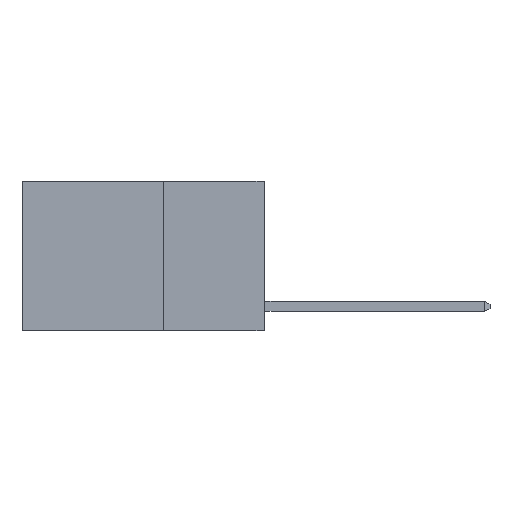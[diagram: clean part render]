
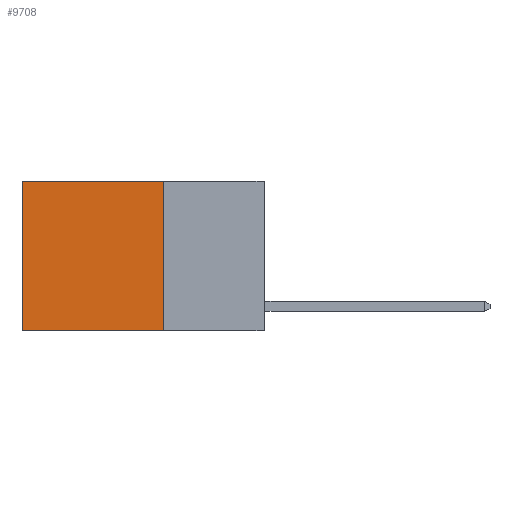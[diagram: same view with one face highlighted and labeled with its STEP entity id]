
A CAD part, left-side view. The second image highlights one B-rep face of the part: STEP entity #9708.
In plain terms, the highlighted planar face has unit normal (-1, 0, 0).
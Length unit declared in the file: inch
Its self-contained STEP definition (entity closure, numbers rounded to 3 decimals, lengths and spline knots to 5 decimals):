
#204 = EDGE_LOOP ( 'NONE', ( #6162, #4687, #380, #394 ) ) ;
#275 = AXIS2_PLACEMENT_3D ( 'NONE', #8043, #2861, #8905 ) ;
#380 = ORIENTED_EDGE ( 'NONE', *, *, #5318, .F. ) ;
#394 = ORIENTED_EDGE ( 'NONE', *, *, #443, .T. ) ;
#443 = EDGE_CURVE ( 'NONE', #10742, #9197, #7298, .T. ) ;
#632 = EDGE_CURVE ( 'NONE', #9197, #9472, #6686, .T. ) ;
#755 = CARTESIAN_POINT ( 'NONE',  ( 0.2625, 0.25, -0.37 ) ) ;
#899 = CARTESIAN_POINT ( 'NONE',  ( 0.2625, 0.6, 0. ) ) ;
#1655 = CARTESIAN_POINT ( 'NONE',  ( 0.2625, 0.6, -0.37 ) ) ;
#2075 = DIRECTION ( 'NONE',  ( 0., 1., 0. ) ) ;
#2601 = CARTESIAN_POINT ( 'NONE',  ( 0.2625, 0.25, 0. ) ) ;
#2861 = DIRECTION ( 'NONE',  ( 1., 0., 0. ) ) ;
#4158 = VECTOR ( 'NONE', #10157, 39.37008 ) ;
#4687 = ORIENTED_EDGE ( 'NONE', *, *, #9145, .F. ) ;
#5124 = LINE ( 'NONE', #2601, #9412 ) ;
#5318 = EDGE_CURVE ( 'NONE', #10742, #5752, #5124, .T. ) ;
#5542 = CARTESIAN_POINT ( 'NONE',  ( 0.2625, 0.25, -0.37 ) ) ;
#5752 = VERTEX_POINT ( 'NONE', #755 ) ;
#6101 = DIRECTION ( 'NONE',  ( 0., 0., -1. ) ) ;
#6162 = ORIENTED_EDGE ( 'NONE', *, *, #632, .T. ) ;
#6234 = CARTESIAN_POINT ( 'NONE',  ( 0.2625, 0.25, 0. ) ) ;
#6686 = LINE ( 'NONE', #899, #11006 ) ;
#7283 = VECTOR ( 'NONE', #2075, 39.37008 ) ;
#7298 = LINE ( 'NONE', #11034, #4158 ) ;
#7403 = FACE_OUTER_BOUND ( 'NONE', #204, .T. ) ;
#8043 = CARTESIAN_POINT ( 'NONE',  ( 0.2625, 0.25, 0. ) ) ;
#8905 = DIRECTION ( 'NONE',  ( 0., 0., -1. ) ) ;
#9145 = EDGE_CURVE ( 'NONE', #5752, #9472, #9290, .T. ) ;
#9197 = VERTEX_POINT ( 'NONE', #9906 ) ;
#9290 = LINE ( 'NONE', #5542, #7283 ) ;
#9412 = VECTOR ( 'NONE', #11256, 39.37008 ) ;
#9472 = VERTEX_POINT ( 'NONE', #1655 ) ;
#9708 = ADVANCED_FACE ( 'NONE', ( #7403 ), #10609, .F. ) ;
#9906 = CARTESIAN_POINT ( 'NONE',  ( 0.2625, 0.6, 0. ) ) ;
#10157 = DIRECTION ( 'NONE',  ( 0., 1., 0. ) ) ;
#10609 = PLANE ( 'NONE',  #275 ) ;
#10742 = VERTEX_POINT ( 'NONE', #6234 ) ;
#11006 = VECTOR ( 'NONE', #6101, 39.37008 ) ;
#11034 = CARTESIAN_POINT ( 'NONE',  ( 0.2625, 0.25, 0. ) ) ;
#11256 = DIRECTION ( 'NONE',  ( 0., 0., -1. ) ) ;
